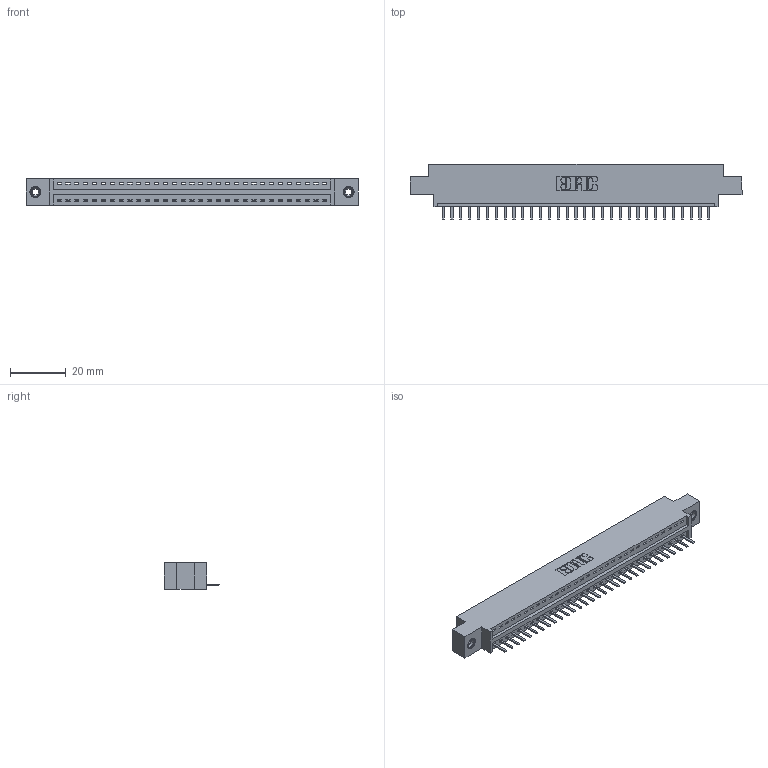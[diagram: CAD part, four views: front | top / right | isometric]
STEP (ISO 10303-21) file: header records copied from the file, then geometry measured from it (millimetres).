
FILE_DESCRIPTION (( 'STEP AP203' ), '1' );
FILE_NAME ('396-031-520-608.STEP', '2018-09-05T08:32:09', ( '' ), ( '' ), 'SwSTEP 2.0', 'SolidWorks 2016', '' );
FILE_SCHEMA (( 'CONFIG_CONTROL_DESIGN' ));
Length unit declared in the file: inch
Products named in the file (4): 345-250-001_345-250-003-102; 396-031-520-608; 346 Part_0.170 Offset - 0.156 Dia-TI; 345-292-001_345-293-120
Assembly tree (34 placements, depth 2):
  396-031-520-608
    346 Part_0.170 Offset - 0.156 Dia-TI
    345-292-001_345-293-120  x31
    345-250-001_345-250-003-102  x2
Bounding box: 119 x 20.02 x 9.4 mm (x, y, z)
Volume: 11064.7 mm3; surface area: 13595.3 mm2
Topology: 34 solids, 34 shells, 2108 faces, 6181 edges, 4030 vertices
Faces by surface type: plane 1414, cylinder 678, cone 12, torus 4
Entity records: 22152 total; most frequent: CARTESIAN_POINT 3796, ORIENTED_EDGE 3742, DIRECTION 3375, EDGE_CURVE 1871, LINE 1591, VECTOR 1591, VERTEX_POINT 1240, AXIS2_PLACEMENT_3D 892
